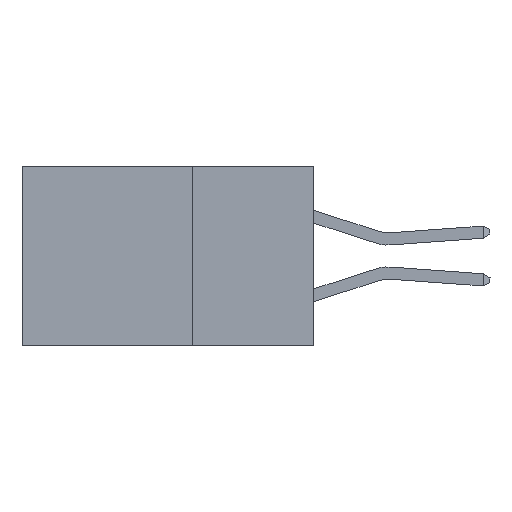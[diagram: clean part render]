
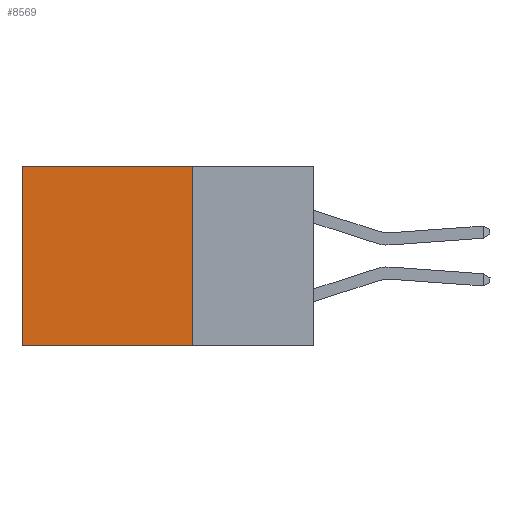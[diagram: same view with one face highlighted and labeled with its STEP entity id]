
A CAD part, left-side view. The second image highlights one B-rep face of the part: STEP entity #8569.
In plain terms, the highlighted planar face has unit normal (-1, 0, 0).
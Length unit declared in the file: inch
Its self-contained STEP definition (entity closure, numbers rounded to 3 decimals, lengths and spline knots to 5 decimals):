
#2181 = CARTESIAN_POINT ( 'NONE',  ( 0.2875, 0.6, 0. ) ) ;
#3075 = ORIENTED_EDGE ( 'NONE', *, *, #22780, .T. ) ;
#3159 = CARTESIAN_POINT ( 'NONE',  ( 0.2875, 0.25, -0.37 ) ) ;
#3333 = CARTESIAN_POINT ( 'NONE',  ( 0.2875, 0.25, 0. ) ) ;
#3529 = VECTOR ( 'NONE', #5798, 39.37008 ) ;
#3599 = VECTOR ( 'NONE', #19581, 39.37008 ) ;
#4676 = CARTESIAN_POINT ( 'NONE',  ( 0.2875, 0.25, -0.37 ) ) ;
#4851 = DIRECTION ( 'NONE',  ( 0., 1., 0. ) ) ;
#5389 = EDGE_LOOP ( 'NONE', ( #3075, #12775, #8439, #18825 ) ) ;
#5429 = LINE ( 'NONE', #2181, #3599 ) ;
#5563 = LINE ( 'NONE', #4676, #16873 ) ;
#5798 = DIRECTION ( 'NONE',  ( 0., 1., 0. ) ) ;
#5886 = DIRECTION ( 'NONE',  ( 0., 0., -1. ) ) ;
#8439 = ORIENTED_EDGE ( 'NONE', *, *, #24180, .F. ) ;
#8569 = ADVANCED_FACE ( 'NONE', ( #10392 ), #8875, .F. ) ;
#8875 = PLANE ( 'NONE',  #19336 ) ;
#10392 = FACE_OUTER_BOUND ( 'NONE', #5389, .T. ) ;
#11007 = DIRECTION ( 'NONE',  ( 1., 0., 0. ) ) ;
#11877 = EDGE_CURVE ( 'NONE', #22341, #23812, #5563, .T. ) ;
#12775 = ORIENTED_EDGE ( 'NONE', *, *, #11877, .F. ) ;
#13301 = VERTEX_POINT ( 'NONE', #18296 ) ;
#13546 = CARTESIAN_POINT ( 'NONE',  ( 0.2875, 0.6, 0. ) ) ;
#13677 = LINE ( 'NONE', #3333, #3529 ) ;
#14873 = EDGE_CURVE ( 'NONE', #13301, #22627, #13677, .T. ) ;
#16267 = CARTESIAN_POINT ( 'NONE',  ( 0.2875, 0.6, -0.37 ) ) ;
#16682 = LINE ( 'NONE', #23383, #16979 ) ;
#16873 = VECTOR ( 'NONE', #4851, 39.37008 ) ;
#16979 = VECTOR ( 'NONE', #5886, 39.37008 ) ;
#18296 = CARTESIAN_POINT ( 'NONE',  ( 0.2875, 0.25, 0. ) ) ;
#18577 = CARTESIAN_POINT ( 'NONE',  ( 0.2875, 0.25, 0. ) ) ;
#18825 = ORIENTED_EDGE ( 'NONE', *, *, #14873, .T. ) ;
#19336 = AXIS2_PLACEMENT_3D ( 'NONE', #18577, #11007, #22854 ) ;
#19581 = DIRECTION ( 'NONE',  ( 0., 0., -1. ) ) ;
#22341 = VERTEX_POINT ( 'NONE', #3159 ) ;
#22627 = VERTEX_POINT ( 'NONE', #13546 ) ;
#22780 = EDGE_CURVE ( 'NONE', #22627, #23812, #5429, .T. ) ;
#22854 = DIRECTION ( 'NONE',  ( 0., 0., -1. ) ) ;
#23383 = CARTESIAN_POINT ( 'NONE',  ( 0.2875, 0.25, 0. ) ) ;
#23812 = VERTEX_POINT ( 'NONE', #16267 ) ;
#24180 = EDGE_CURVE ( 'NONE', #13301, #22341, #16682, .T. ) ;
